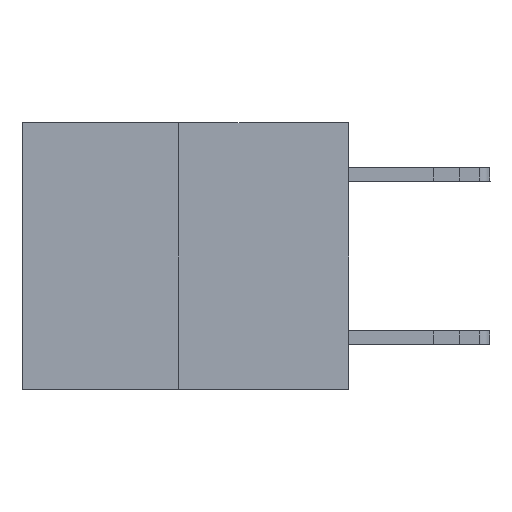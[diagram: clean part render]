
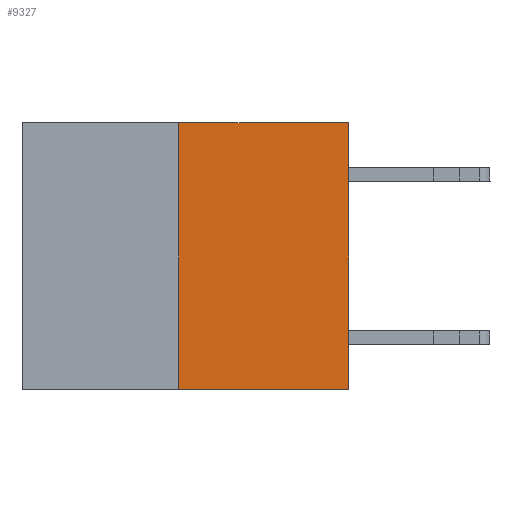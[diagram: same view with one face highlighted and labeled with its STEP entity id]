
A CAD part, left-side view. The second image highlights one B-rep face of the part: STEP entity #9327.
In plain terms, the highlighted planar face has unit normal (-1, 0, 0).
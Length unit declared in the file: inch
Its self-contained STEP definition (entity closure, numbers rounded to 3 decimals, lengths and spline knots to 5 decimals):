
#41 = DIRECTION ( 'NONE',  ( 0., 0., 1. ) ) ;
#227 = LINE ( 'NONE', #28389, #25123 ) ;
#1724 = PLANE ( 'NONE',  #30391 ) ;
#2403 = FACE_OUTER_BOUND ( 'NONE', #29352, .T. ) ;
#3965 = CARTESIAN_POINT ( 'NONE',  ( 0., 0.6, -0.49 ) ) ;
#5684 = EDGE_CURVE ( 'NONE', #19818, #7987, #8411, .T. ) ;
#5983 = CARTESIAN_POINT ( 'NONE',  ( 0., 0.312, -0.49 ) ) ;
#6129 = VERTEX_POINT ( 'NONE', #5983 ) ;
#6297 = EDGE_CURVE ( 'NONE', #16733, #7987, #26199, .T. ) ;
#6745 = ORIENTED_EDGE ( 'NONE', *, *, #21785, .F. ) ;
#7116 = CARTESIAN_POINT ( 'NONE',  ( 0., 0.6, 0. ) ) ;
#7252 = DIRECTION ( 'NONE',  ( 0., 0., -1. ) ) ;
#7987 = VERTEX_POINT ( 'NONE', #21801 ) ;
#8115 = VECTOR ( 'NONE', #11027, 39.37008 ) ;
#8411 = LINE ( 'NONE', #11390, #29162 ) ;
#8755 = ORIENTED_EDGE ( 'NONE', *, *, #5684, .T. ) ;
#9327 = ADVANCED_FACE ( 'NONE', ( #2403 ), #1724, .F. ) ;
#11027 = DIRECTION ( 'NONE',  ( 0., -1., 0. ) ) ;
#11390 = CARTESIAN_POINT ( 'NONE',  ( 0., 0., 0. ) ) ;
#12083 = DIRECTION ( 'NONE',  ( 0., -1., 0. ) ) ;
#13509 = EDGE_CURVE ( 'NONE', #6129, #19818, #19262, .T. ) ;
#16683 = ORIENTED_EDGE ( 'NONE', *, *, #13509, .T. ) ;
#16733 = VERTEX_POINT ( 'NONE', #28226 ) ;
#18969 = CARTESIAN_POINT ( 'NONE',  ( 0., 0.6, 0. ) ) ;
#19262 = LINE ( 'NONE', #3965, #8115 ) ;
#19818 = VERTEX_POINT ( 'NONE', #22457 ) ;
#21246 = DIRECTION ( 'NONE',  ( 1., 0., 0. ) ) ;
#21785 = EDGE_CURVE ( 'NONE', #6129, #16733, #227, .T. ) ;
#21801 = CARTESIAN_POINT ( 'NONE',  ( 0., 0., 0. ) ) ;
#22457 = CARTESIAN_POINT ( 'NONE',  ( 0., 0., -0.49 ) ) ;
#23957 = VECTOR ( 'NONE', #12083, 39.37008 ) ;
#25123 = VECTOR ( 'NONE', #41, 39.37008 ) ;
#26035 = DIRECTION ( 'NONE',  ( 0., 0., 1. ) ) ;
#26199 = LINE ( 'NONE', #7116, #23957 ) ;
#26904 = ORIENTED_EDGE ( 'NONE', *, *, #6297, .F. ) ;
#28226 = CARTESIAN_POINT ( 'NONE',  ( 0., 0.312, 0. ) ) ;
#28389 = CARTESIAN_POINT ( 'NONE',  ( 0., 0.312, -0.49 ) ) ;
#29162 = VECTOR ( 'NONE', #26035, 39.37008 ) ;
#29352 = EDGE_LOOP ( 'NONE', ( #6745, #16683, #8755, #26904 ) ) ;
#30391 = AXIS2_PLACEMENT_3D ( 'NONE', #18969, #21246, #7252 ) ;
